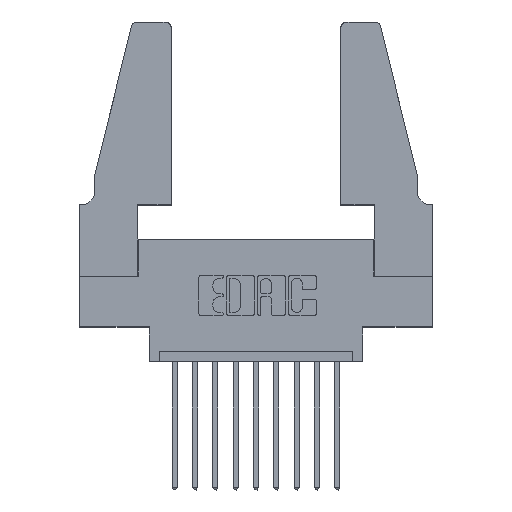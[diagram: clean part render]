
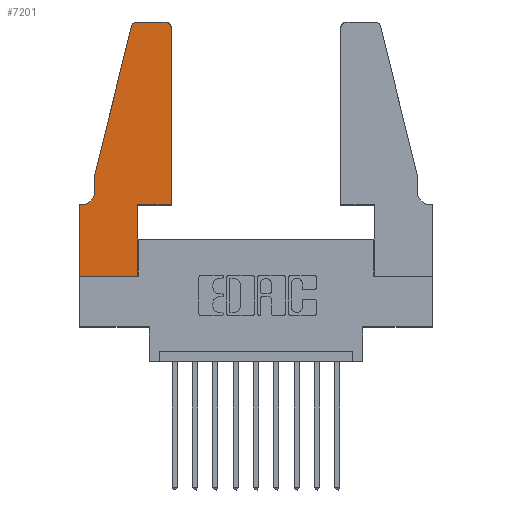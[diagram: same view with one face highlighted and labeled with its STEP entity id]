
A CAD part, top view. The second image highlights one B-rep face of the part: STEP entity #7201.
In plain terms, the highlighted planar face has unit normal (0, 0, 1).
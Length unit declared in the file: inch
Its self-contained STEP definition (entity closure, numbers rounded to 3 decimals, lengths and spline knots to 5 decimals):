
#85 = AXIS2_PLACEMENT_3D ( 'NONE', #1014, #3147, #10453 ) ;
#511 = CARTESIAN_POINT ( 'NONE',  ( 0.0755, 0.5, 0.37 ) ) ;
#524 = ORIENTED_EDGE ( 'NONE', *, *, #1761, .T. ) ;
#598 = CARTESIAN_POINT ( 'NONE',  ( 0.0755, 0.5, 0.37 ) ) ;
#611 = PLANE ( 'NONE',  #5202 ) ;
#741 = ORIENTED_EDGE ( 'NONE', *, *, #10549, .T. ) ;
#998 = CARTESIAN_POINT ( 'NONE',  ( 0.4505, 0.35, 0.37 ) ) ;
#1014 = CARTESIAN_POINT ( 'NONE',  ( 0.0055, 0.42, 0.37 ) ) ;
#1431 = DIRECTION ( 'NONE',  ( 0., 0., 1. ) ) ;
#1761 = EDGE_CURVE ( 'NONE', #7666, #1776, #12123, .T. ) ;
#1776 = VERTEX_POINT ( 'NONE', #4234 ) ;
#1985 = CARTESIAN_POINT ( 'NONE',  ( 0.0755, 0.42, 0.37 ) ) ;
#2245 = ORIENTED_EDGE ( 'NONE', *, *, #11987, .T. ) ;
#2519 = LINE ( 'NONE', #13464, #4492 ) ;
#2554 = ORIENTED_EDGE ( 'NONE', *, *, #8545, .T. ) ;
#2634 = LINE ( 'NONE', #4129, #3624 ) ;
#2703 = VECTOR ( 'NONE', #13161, 39.37008 ) ;
#2725 = DIRECTION ( 'NONE',  ( 0., 0., 1. ) ) ;
#2770 = VERTEX_POINT ( 'NONE', #6541 ) ;
#2810 = ORIENTED_EDGE ( 'NONE', *, *, #11725, .T. ) ;
#2951 = CARTESIAN_POINT ( 'NONE',  ( 0.2865, 0.35, 0.37 ) ) ;
#2990 = DIRECTION ( 'NONE',  ( 0., 1., 0. ) ) ;
#3091 = ORIENTED_EDGE ( 'NONE', *, *, #6526, .T. ) ;
#3138 = LINE ( 'NONE', #998, #12596 ) ;
#3147 = DIRECTION ( 'NONE',  ( 0., 0., -1. ) ) ;
#3168 = VERTEX_POINT ( 'NONE', #10366 ) ;
#3300 = LINE ( 'NONE', #12753, #10990 ) ;
#3404 = CARTESIAN_POINT ( 'NONE',  ( 0.4205, 1.22, 0.37 ) ) ;
#3513 = ORIENTED_EDGE ( 'NONE', *, *, #13292, .T. ) ;
#3624 = VECTOR ( 'NONE', #12327, 39.37008 ) ;
#3734 = DIRECTION ( 'NONE',  ( -0.239, -0.971, 0. ) ) ;
#3976 = VECTOR ( 'NONE', #8560, 39.37008 ) ;
#4003 = CARTESIAN_POINT ( 'NONE',  ( 0.284, 1.22, 0.37 ) ) ;
#4129 = CARTESIAN_POINT ( 'NONE',  ( 0., 0., 0.37 ) ) ;
#4234 = CARTESIAN_POINT ( 'NONE',  ( 0., 0.35, 0.37 ) ) ;
#4304 = EDGE_CURVE ( 'NONE', #9087, #10279, #8142, .T. ) ;
#4305 = CARTESIAN_POINT ( 'NONE',  ( 0.2865, 0.35, 0.37 ) ) ;
#4492 = VECTOR ( 'NONE', #7185, 39.37008 ) ;
#4989 = VERTEX_POINT ( 'NONE', #12236 ) ;
#5202 = AXIS2_PLACEMENT_3D ( 'NONE', #7948, #2725, #12186 ) ;
#5342 = VERTEX_POINT ( 'NONE', #4305 ) ;
#6115 = FACE_OUTER_BOUND ( 'NONE', #7207, .T. ) ;
#6150 = DIRECTION ( 'NONE',  ( 0., 0., 1. ) ) ;
#6526 = EDGE_CURVE ( 'NONE', #4989, #9087, #7115, .T. ) ;
#6541 = CARTESIAN_POINT ( 'NONE',  ( 0.4505, 0.35, 0.37 ) ) ;
#6558 = VECTOR ( 'NONE', #12289, 39.37008 ) ;
#6635 = CIRCLE ( 'NONE', #85, 0.07 ) ;
#6686 = DIRECTION ( 'NONE',  ( 1., 0., 0. ) ) ;
#7115 = CIRCLE ( 'NONE', #12269, 0.03 ) ;
#7185 = DIRECTION ( 'NONE',  ( 0., -1., 0. ) ) ;
#7201 = ADVANCED_FACE ( 'NONE', ( #6115 ), #611, .T. ) ;
#7207 = EDGE_LOOP ( 'NONE', ( #2554, #3091, #8419, #2810, #2245, #524, #13534, #13450, #13283, #3513, #8284, #741 ) ) ;
#7471 = CARTESIAN_POINT ( 'NONE',  ( 0.4505, 1.22, 0.37 ) ) ;
#7495 = VECTOR ( 'NONE', #3734, 39.37008 ) ;
#7666 = VERTEX_POINT ( 'NONE', #12879 ) ;
#7686 = LINE ( 'NONE', #8407, #6558 ) ;
#7882 = EDGE_CURVE ( 'NONE', #3168, #9802, #2634, .T. ) ;
#7948 = CARTESIAN_POINT ( 'NONE',  ( 0., 0.35, 0.37 ) ) ;
#8057 = CARTESIAN_POINT ( 'NONE',  ( 0.25487, 1.22718, 0.37 ) ) ;
#8098 = LINE ( 'NONE', #511, #2703 ) ;
#8142 = LINE ( 'NONE', #598, #7495 ) ;
#8284 = ORIENTED_EDGE ( 'NONE', *, *, #12953, .T. ) ;
#8407 = CARTESIAN_POINT ( 'NONE',  ( 0.2605, 1.25, 0.37 ) ) ;
#8419 = ORIENTED_EDGE ( 'NONE', *, *, #4304, .T. ) ;
#8545 = EDGE_CURVE ( 'NONE', #9133, #4989, #7686, .T. ) ;
#8560 = DIRECTION ( 'NONE',  ( -1., 0., 0. ) ) ;
#9087 = VERTEX_POINT ( 'NONE', #8057 ) ;
#9133 = VERTEX_POINT ( 'NONE', #10188 ) ;
#9802 = VERTEX_POINT ( 'NONE', #13324 ) ;
#10188 = CARTESIAN_POINT ( 'NONE',  ( 0.4205, 1.25, 0.37 ) ) ;
#10279 = VERTEX_POINT ( 'NONE', #11174 ) ;
#10366 = CARTESIAN_POINT ( 'NONE',  ( 0., 0., 0.37 ) ) ;
#10453 = DIRECTION ( 'NONE',  ( -1., 0., 0. ) ) ;
#10488 = VECTOR ( 'NONE', #12354, 39.37008 ) ;
#10549 = EDGE_CURVE ( 'NONE', #10967, #9133, #12523, .T. ) ;
#10967 = VERTEX_POINT ( 'NONE', #7471 ) ;
#10990 = VECTOR ( 'NONE', #11814, 39.37008 ) ;
#11174 = CARTESIAN_POINT ( 'NONE',  ( 0.0755, 0.5, 0.37 ) ) ;
#11235 = AXIS2_PLACEMENT_3D ( 'NONE', #3404, #1431, #6686 ) ;
#11300 = DIRECTION ( 'NONE',  ( 1., 0., 0. ) ) ;
#11512 = CARTESIAN_POINT ( 'NONE',  ( 0.0755, 0.35, 0.37 ) ) ;
#11725 = EDGE_CURVE ( 'NONE', #10279, #13172, #8098, .T. ) ;
#11814 = DIRECTION ( 'NONE',  ( 1., 0., 0. ) ) ;
#11987 = EDGE_CURVE ( 'NONE', #13172, #7666, #6635, .T. ) ;
#12123 = LINE ( 'NONE', #11512, #3976 ) ;
#12186 = DIRECTION ( 'NONE',  ( 1., 0., 0. ) ) ;
#12236 = CARTESIAN_POINT ( 'NONE',  ( 0.284, 1.25, 0.37 ) ) ;
#12269 = AXIS2_PLACEMENT_3D ( 'NONE', #4003, #6150, #11300 ) ;
#12289 = DIRECTION ( 'NONE',  ( -1., 0., 0. ) ) ;
#12293 = LINE ( 'NONE', #2951, #10488 ) ;
#12327 = DIRECTION ( 'NONE',  ( 1., 0., 0. ) ) ;
#12354 = DIRECTION ( 'NONE',  ( 0., 1., 0. ) ) ;
#12422 = EDGE_CURVE ( 'NONE', #1776, #3168, #2519, .T. ) ;
#12523 = CIRCLE ( 'NONE', #11235, 0.03 ) ;
#12596 = VECTOR ( 'NONE', #2990, 39.37008 ) ;
#12753 = CARTESIAN_POINT ( 'NONE',  ( 0.4505, 0.35, 0.37 ) ) ;
#12879 = CARTESIAN_POINT ( 'NONE',  ( 0.0055, 0.35, 0.37 ) ) ;
#12953 = EDGE_CURVE ( 'NONE', #2770, #10967, #3138, .T. ) ;
#13122 = EDGE_CURVE ( 'NONE', #9802, #5342, #12293, .T. ) ;
#13161 = DIRECTION ( 'NONE',  ( 0., -1., 0. ) ) ;
#13172 = VERTEX_POINT ( 'NONE', #1985 ) ;
#13283 = ORIENTED_EDGE ( 'NONE', *, *, #13122, .T. ) ;
#13292 = EDGE_CURVE ( 'NONE', #5342, #2770, #3300, .T. ) ;
#13324 = CARTESIAN_POINT ( 'NONE',  ( 0.2865, 0., 0.37 ) ) ;
#13450 = ORIENTED_EDGE ( 'NONE', *, *, #7882, .T. ) ;
#13464 = CARTESIAN_POINT ( 'NONE',  ( 0., 0., 0.37 ) ) ;
#13534 = ORIENTED_EDGE ( 'NONE', *, *, #12422, .T. ) ;
